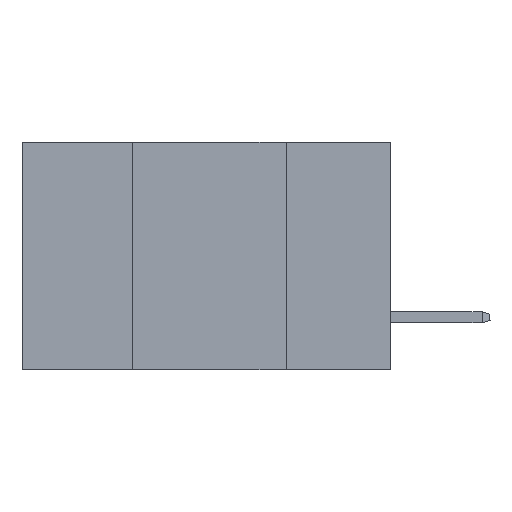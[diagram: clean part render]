
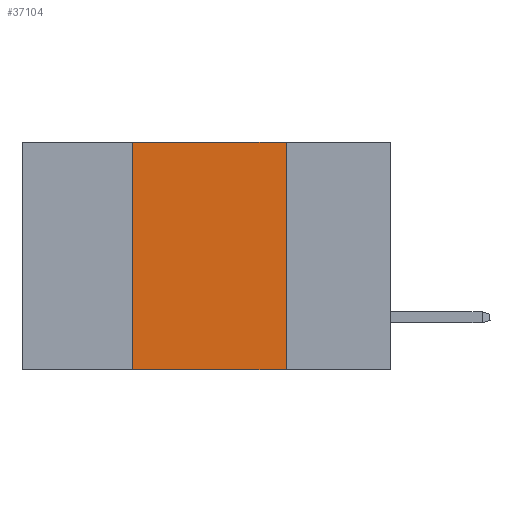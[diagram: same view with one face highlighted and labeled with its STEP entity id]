
A CAD part, left-side view. The second image highlights one B-rep face of the part: STEP entity #37104.
In plain terms, the highlighted planar face has unit normal (-1, 0, 0).
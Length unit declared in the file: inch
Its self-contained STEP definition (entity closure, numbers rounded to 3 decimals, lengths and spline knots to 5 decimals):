
#63 = VERTEX_POINT ( 'NONE', #47699 ) ;
#976 = LINE ( 'NONE', #32494, #31999 ) ;
#1181 = EDGE_CURVE ( 'NONE', #47361, #63, #28901, .T. ) ;
#1850 = EDGE_LOOP ( 'NONE', ( #32757, #17610, #27281, #27118 ) ) ;
#3164 = EDGE_CURVE ( 'NONE', #63, #26044, #12678, .T. ) ;
#3500 = DIRECTION ( 'NONE',  ( 0., 0., -1. ) ) ;
#7104 = EDGE_CURVE ( 'NONE', #47361, #7428, #45754, .T. ) ;
#7428 = VERTEX_POINT ( 'NONE', #42333 ) ;
#9172 = EDGE_CURVE ( 'NONE', #26044, #7428, #976, .T. ) ;
#12678 = LINE ( 'NONE', #30420, #47359 ) ;
#14510 = DIRECTION ( 'NONE',  ( 0., 0., 1. ) ) ;
#14830 = AXIS2_PLACEMENT_3D ( 'NONE', #38361, #41906, #3500 ) ;
#17610 = ORIENTED_EDGE ( 'NONE', *, *, #3164, .F. ) ;
#18541 = VECTOR ( 'NONE', #14510, 39.37008 ) ;
#25354 = DIRECTION ( 'NONE',  ( 0., 0., -1. ) ) ;
#26044 = VERTEX_POINT ( 'NONE', #46436 ) ;
#26468 = PLANE ( 'NONE',  #14830 ) ;
#27118 = ORIENTED_EDGE ( 'NONE', *, *, #7104, .T. ) ;
#27281 = ORIENTED_EDGE ( 'NONE', *, *, #1181, .F. ) ;
#28786 = CARTESIAN_POINT ( 'NONE',  ( 0., 0.6, -0.37 ) ) ;
#28901 = LINE ( 'NONE', #46273, #18541 ) ;
#30420 = CARTESIAN_POINT ( 'NONE',  ( 0., 0.6, 0. ) ) ;
#31999 = VECTOR ( 'NONE', #25354, 39.37008 ) ;
#32494 = CARTESIAN_POINT ( 'NONE',  ( 0., 0.17, 0. ) ) ;
#32757 = ORIENTED_EDGE ( 'NONE', *, *, #9172, .F. ) ;
#37104 = ADVANCED_FACE ( 'NONE', ( #41205 ), #26468, .F. ) ;
#38361 = CARTESIAN_POINT ( 'NONE',  ( 0., 0.6, 0. ) ) ;
#39042 = CARTESIAN_POINT ( 'NONE',  ( 0., 0.42, -0.37 ) ) ;
#39823 = DIRECTION ( 'NONE',  ( 0., -1., 0. ) ) ;
#41059 = DIRECTION ( 'NONE',  ( 0., -1., 0. ) ) ;
#41205 = FACE_OUTER_BOUND ( 'NONE', #1850, .T. ) ;
#41906 = DIRECTION ( 'NONE',  ( 1., 0., 0. ) ) ;
#42114 = VECTOR ( 'NONE', #39823, 39.37008 ) ;
#42333 = CARTESIAN_POINT ( 'NONE',  ( 0., 0.17, -0.37 ) ) ;
#45754 = LINE ( 'NONE', #28786, #42114 ) ;
#46273 = CARTESIAN_POINT ( 'NONE',  ( 0., 0.42, 0. ) ) ;
#46436 = CARTESIAN_POINT ( 'NONE',  ( 0., 0.17, 0. ) ) ;
#47359 = VECTOR ( 'NONE', #41059, 39.37008 ) ;
#47361 = VERTEX_POINT ( 'NONE', #39042 ) ;
#47699 = CARTESIAN_POINT ( 'NONE',  ( 0., 0.42, 0. ) ) ;
